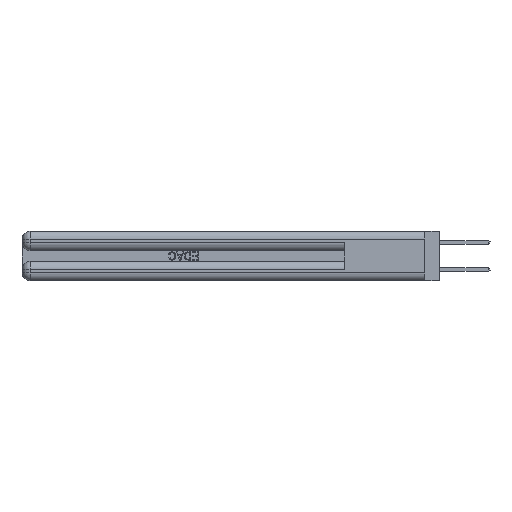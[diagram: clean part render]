
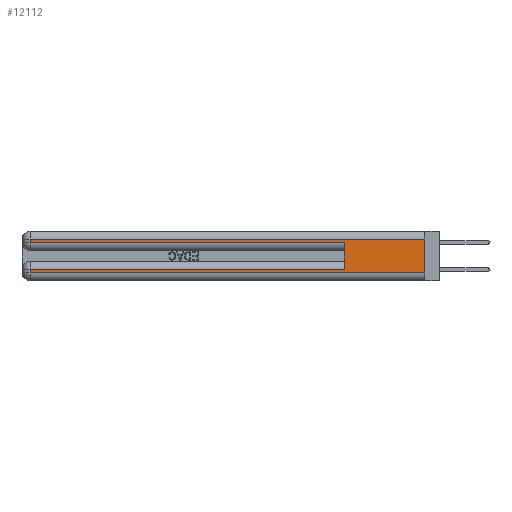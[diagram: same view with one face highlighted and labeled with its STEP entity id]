
A CAD part, left-side view. The second image highlights one B-rep face of the part: STEP entity #12112.
In plain terms, the highlighted planar face has unit normal (-1, 0, 0).
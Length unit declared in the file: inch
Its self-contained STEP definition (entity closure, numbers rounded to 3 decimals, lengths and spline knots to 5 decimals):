
#4 = CARTESIAN_POINT ( 'NONE',  ( 0., 2.94, 0.285 ) ) ;
#597 = CARTESIAN_POINT ( 'NONE',  ( 0., 0., 0.06 ) ) ;
#859 = VERTEX_POINT ( 'NONE', #17434 ) ;
#987 = DIRECTION ( 'NONE',  ( 1., 0., 0. ) ) ;
#1218 = VERTEX_POINT ( 'NONE', #597 ) ;
#1385 = DIRECTION ( 'NONE',  ( 0., 0., -1. ) ) ;
#3480 = ORIENTED_EDGE ( 'NONE', *, *, #9225, .T. ) ;
#3665 = ORIENTED_EDGE ( 'NONE', *, *, #34953, .T. ) ;
#3885 = VECTOR ( 'NONE', #8153, 39.37008 ) ;
#4221 = EDGE_CURVE ( 'NONE', #13577, #27509, #15132, .T. ) ;
#5070 = VECTOR ( 'NONE', #37596, 39.37008 ) ;
#5417 = ORIENTED_EDGE ( 'NONE', *, *, #10194, .T. ) ;
#6575 = CARTESIAN_POINT ( 'NONE',  ( 0., 2.94, 0.37 ) ) ;
#6735 = ORIENTED_EDGE ( 'NONE', *, *, #37139, .F. ) ;
#7257 = VERTEX_POINT ( 'NONE', #31441 ) ;
#7851 = CARTESIAN_POINT ( 'NONE',  ( 0., 0.6, 0.145 ) ) ;
#8153 = DIRECTION ( 'NONE',  ( 0., 0., 1. ) ) ;
#9225 = EDGE_CURVE ( 'NONE', #7257, #37236, #13518, .T. ) ;
#9256 = VECTOR ( 'NONE', #31693, 39.37008 ) ;
#9496 = VECTOR ( 'NONE', #11609, 39.37008 ) ;
#9654 = EDGE_CURVE ( 'NONE', #27509, #19530, #43429, .T. ) ;
#10194 = EDGE_CURVE ( 'NONE', #19530, #859, #33324, .T. ) ;
#10725 = DIRECTION ( 'NONE',  ( 0., 1., 0. ) ) ;
#11609 = DIRECTION ( 'NONE',  ( 0., 1., 0. ) ) ;
#12112 = ADVANCED_FACE ( 'NONE', ( #26850 ), #31423, .F. ) ;
#13518 = LINE ( 'NONE', #6575, #5070 ) ;
#13577 = VERTEX_POINT ( 'NONE', #28870 ) ;
#13822 = VERTEX_POINT ( 'NONE', #19221 ) ;
#14603 = LINE ( 'NONE', #40817, #40352 ) ;
#15015 = ORIENTED_EDGE ( 'NONE', *, *, #20526, .F. ) ;
#15132 = LINE ( 'NONE', #31989, #42990 ) ;
#17434 = CARTESIAN_POINT ( 'NONE',  ( 0., 0.6, 0.285 ) ) ;
#17580 = CARTESIAN_POINT ( 'NONE',  ( 0., 2.94, 0.37 ) ) ;
#18121 = CARTESIAN_POINT ( 'NONE',  ( 0., 0., 0.37 ) ) ;
#19221 = CARTESIAN_POINT ( 'NONE',  ( 0., 0.6, 0.085 ) ) ;
#19530 = VERTEX_POINT ( 'NONE', #4 ) ;
#19833 = ORIENTED_EDGE ( 'NONE', *, *, #33367, .T. ) ;
#20526 = EDGE_CURVE ( 'NONE', #13577, #1218, #25004, .T. ) ;
#20807 = EDGE_LOOP ( 'NONE', ( #15015, #35026, #37322, #5417, #6735, #19833, #3480, #3665 ) ) ;
#22318 = LINE ( 'NONE', #7851, #3885 ) ;
#23367 = CARTESIAN_POINT ( 'NONE',  ( 0., 0., 0.285 ) ) ;
#25004 = LINE ( 'NONE', #18121, #31301 ) ;
#25409 = CARTESIAN_POINT ( 'NONE',  ( 0., 0., 0.085 ) ) ;
#26718 = DIRECTION ( 'NONE',  ( 0., -1., 0. ) ) ;
#26850 = FACE_OUTER_BOUND ( 'NONE', #20807, .T. ) ;
#27509 = VERTEX_POINT ( 'NONE', #28136 ) ;
#27738 = DIRECTION ( 'NONE',  ( 0., -1., 0. ) ) ;
#28136 = CARTESIAN_POINT ( 'NONE',  ( 0., 2.94, 0.31 ) ) ;
#28870 = CARTESIAN_POINT ( 'NONE',  ( 0., 0., 0.31 ) ) ;
#31301 = VECTOR ( 'NONE', #1385, 39.37008 ) ;
#31423 = PLANE ( 'NONE',  #38009 ) ;
#31441 = CARTESIAN_POINT ( 'NONE',  ( 0., 2.94, 0.085 ) ) ;
#31693 = DIRECTION ( 'NONE',  ( 0., 0., -1. ) ) ;
#31989 = CARTESIAN_POINT ( 'NONE',  ( 0., 0., 0.31 ) ) ;
#33324 = LINE ( 'NONE', #23367, #34338 ) ;
#33367 = EDGE_CURVE ( 'NONE', #13822, #7257, #41003, .T. ) ;
#34338 = VECTOR ( 'NONE', #26718, 39.37008 ) ;
#34697 = CARTESIAN_POINT ( 'NONE',  ( 0., 2.94, 0.06 ) ) ;
#34953 = EDGE_CURVE ( 'NONE', #37236, #1218, #14603, .T. ) ;
#35026 = ORIENTED_EDGE ( 'NONE', *, *, #4221, .T. ) ;
#37139 = EDGE_CURVE ( 'NONE', #13822, #859, #22318, .T. ) ;
#37236 = VERTEX_POINT ( 'NONE', #34697 ) ;
#37322 = ORIENTED_EDGE ( 'NONE', *, *, #9654, .T. ) ;
#37596 = DIRECTION ( 'NONE',  ( 0., 0., -1. ) ) ;
#38009 = AXIS2_PLACEMENT_3D ( 'NONE', #41271, #987, #38155 ) ;
#38155 = DIRECTION ( 'NONE',  ( 0., 0., -1. ) ) ;
#40352 = VECTOR ( 'NONE', #27738, 39.37008 ) ;
#40817 = CARTESIAN_POINT ( 'NONE',  ( 0., 0., 0.06 ) ) ;
#41003 = LINE ( 'NONE', #25409, #9496 ) ;
#41271 = CARTESIAN_POINT ( 'NONE',  ( 0., 0., 0.37 ) ) ;
#42990 = VECTOR ( 'NONE', #10725, 39.37008 ) ;
#43429 = LINE ( 'NONE', #17580, #9256 ) ;
